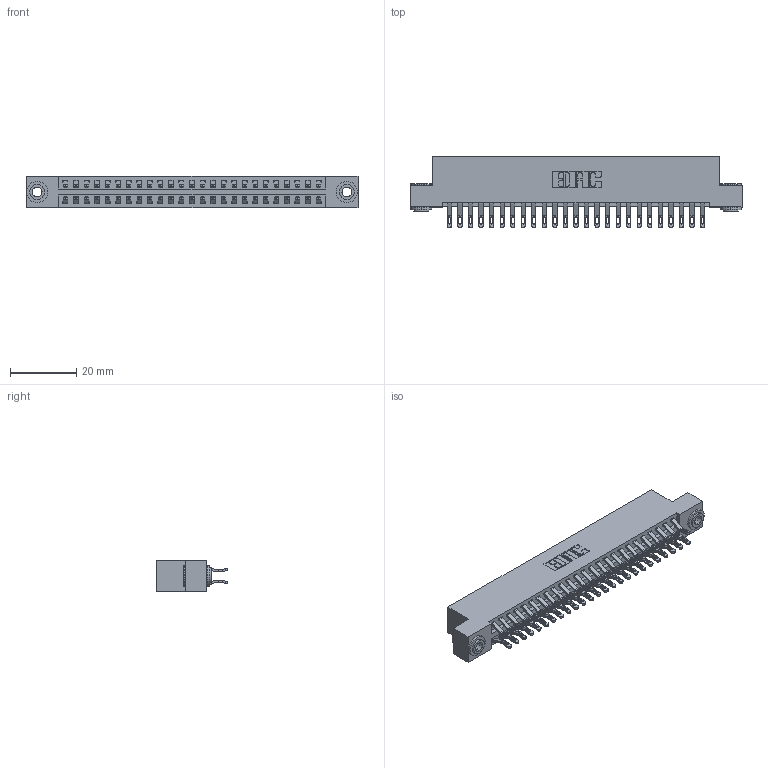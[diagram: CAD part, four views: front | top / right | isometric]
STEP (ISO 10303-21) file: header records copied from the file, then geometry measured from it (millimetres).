
FILE_DESCRIPTION (( 'STEP AP203' ), '1' );
FILE_NAME ('346-050-555-203.STEP', '2022-05-20T23:34:57', ( '' ), ( '' ), 'SwSTEP 2.0', 'SolidWorks 2020', '' );
FILE_SCHEMA (( 'CONFIG_CONTROL_DESIGN' ));
Length unit declared in the file: inch
Products named in the file (4): 345-292-001_555 Tail; 346-050-555-203; 345-250-002_345-250-002-102; 346 Part_Flush Mounting Lugs - 0.156 Dia-TH
Assembly tree (53 placements, depth 2):
  346-050-555-203
    346 Part_Flush Mounting Lugs - 0.156 Dia-TH
    345-292-001_555 Tail  x50
    345-250-002_345-250-002-102  x2
Bounding box: 99.95 x 21.46 x 9.4 mm (x, y, z)
Volume: 9760.6 mm3; surface area: 13915 mm2
Topology: 53 solids, 53 shells, 3074 faces, 9591 edges, 6390 vertices
Faces by surface type: plane 1750, cylinder 1316, cone 8
Entity records: 19996 total; most frequent: CARTESIAN_POINT 3335, ORIENTED_EDGE 3230, DIRECTION 2989, EDGE_CURVE 1615, LINE 1339, VECTOR 1339, VERTEX_POINT 1074, AXIS2_PLACEMENT_3D 825
